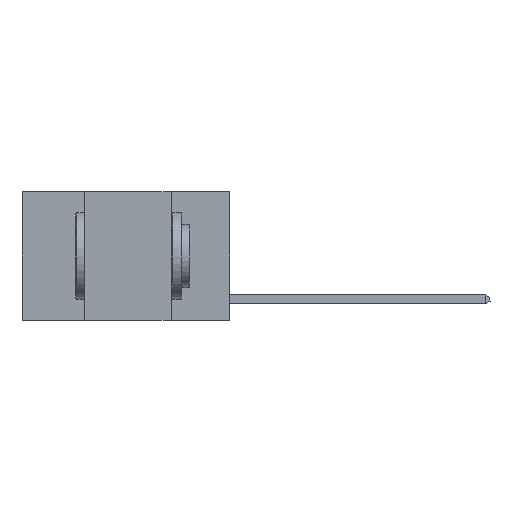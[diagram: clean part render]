
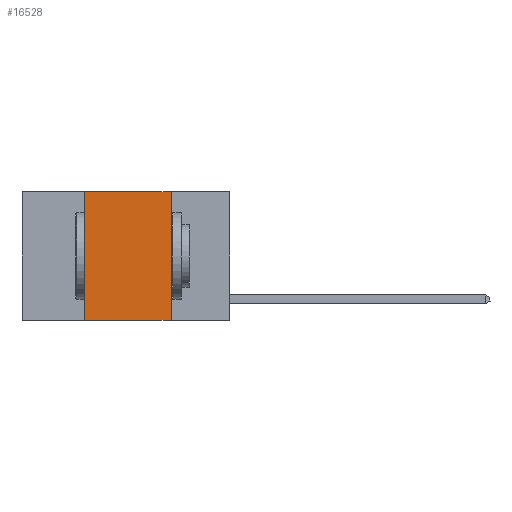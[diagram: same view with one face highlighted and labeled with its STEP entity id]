
A CAD part, left-side view. The second image highlights one B-rep face of the part: STEP entity #16528.
In plain terms, the highlighted planar face has unit normal (-1, 0, 0).
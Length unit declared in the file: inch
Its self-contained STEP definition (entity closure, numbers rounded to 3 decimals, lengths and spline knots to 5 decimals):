
#335 = FACE_OUTER_BOUND ( 'NONE', #10576, .T. ) ;
#439 = CARTESIAN_POINT ( 'NONE',  ( 0., 0.42, 0. ) ) ;
#688 = PLANE ( 'NONE',  #14508 ) ;
#1494 = VERTEX_POINT ( 'NONE', #8084 ) ;
#1740 = CARTESIAN_POINT ( 'NONE',  ( 0., 0.42, 0. ) ) ;
#2610 = CARTESIAN_POINT ( 'NONE',  ( 0., 0.42, -0.37 ) ) ;
#4251 = EDGE_CURVE ( 'NONE', #6740, #15194, #9911, .T. ) ;
#4361 = EDGE_CURVE ( 'NONE', #14724, #1494, #8057, .T. ) ;
#5075 = VECTOR ( 'NONE', #9282, 39.37008 ) ;
#5122 = CARTESIAN_POINT ( 'NONE',  ( 0., 0.6, 0. ) ) ;
#6198 = DIRECTION ( 'NONE',  ( 0., -1., 0. ) ) ;
#6611 = CARTESIAN_POINT ( 'NONE',  ( 0., 0.6, -0.37 ) ) ;
#6740 = VERTEX_POINT ( 'NONE', #1740 ) ;
#7466 = ORIENTED_EDGE ( 'NONE', *, *, #4251, .F. ) ;
#7536 = DIRECTION ( 'NONE',  ( 0., -1., 0. ) ) ;
#7572 = CARTESIAN_POINT ( 'NONE',  ( 0., 0.6, 0. ) ) ;
#8057 = LINE ( 'NONE', #6611, #15410 ) ;
#8084 = CARTESIAN_POINT ( 'NONE',  ( 0., 0.17, -0.37 ) ) ;
#8924 = CARTESIAN_POINT ( 'NONE',  ( 0., 0.17, 0. ) ) ;
#9282 = DIRECTION ( 'NONE',  ( 0., 0., 1. ) ) ;
#9610 = DIRECTION ( 'NONE',  ( 0., 0., -1. ) ) ;
#9911 = LINE ( 'NONE', #7572, #17295 ) ;
#10464 = DIRECTION ( 'NONE',  ( 0., 0., -1. ) ) ;
#10576 = EDGE_LOOP ( 'NONE', ( #12314, #7466, #14172, #10814 ) ) ;
#10814 = ORIENTED_EDGE ( 'NONE', *, *, #4361, .T. ) ;
#12314 = ORIENTED_EDGE ( 'NONE', *, *, #17085, .F. ) ;
#14172 = ORIENTED_EDGE ( 'NONE', *, *, #14456, .F. ) ;
#14456 = EDGE_CURVE ( 'NONE', #14724, #6740, #17294, .T. ) ;
#14508 = AXIS2_PLACEMENT_3D ( 'NONE', #5122, #18429, #9610 ) ;
#14724 = VERTEX_POINT ( 'NONE', #2610 ) ;
#15194 = VERTEX_POINT ( 'NONE', #16880 ) ;
#15410 = VECTOR ( 'NONE', #6198, 39.37008 ) ;
#16528 = ADVANCED_FACE ( 'NONE', ( #335 ), #688, .F. ) ;
#16880 = CARTESIAN_POINT ( 'NONE',  ( 0., 0.17, 0. ) ) ;
#17085 = EDGE_CURVE ( 'NONE', #15194, #1494, #17636, .T. ) ;
#17185 = VECTOR ( 'NONE', #10464, 39.37008 ) ;
#17294 = LINE ( 'NONE', #439, #5075 ) ;
#17295 = VECTOR ( 'NONE', #7536, 39.37008 ) ;
#17636 = LINE ( 'NONE', #8924, #17185 ) ;
#18429 = DIRECTION ( 'NONE',  ( 1., 0., 0. ) ) ;
